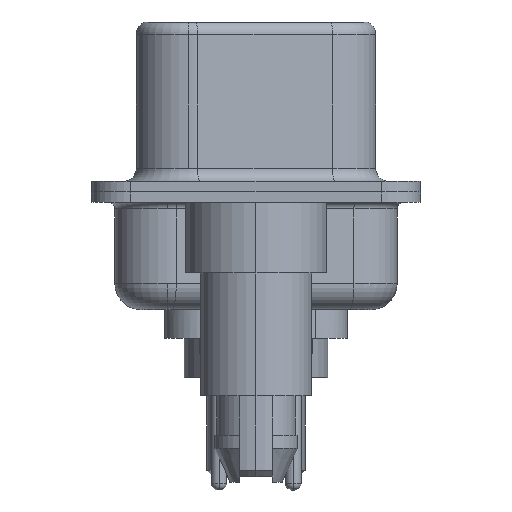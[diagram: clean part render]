
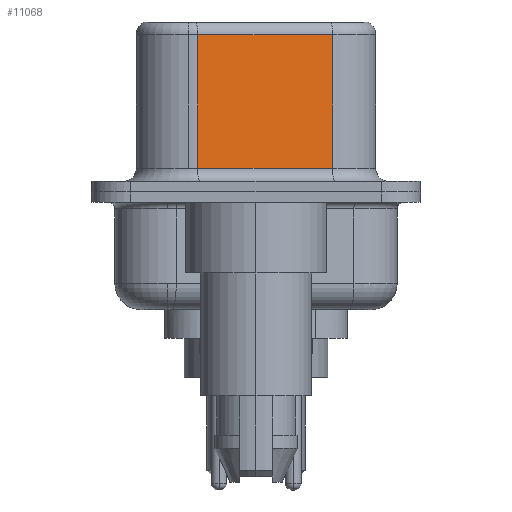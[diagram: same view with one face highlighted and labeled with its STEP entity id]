
A CAD part, left-side view. The second image highlights one B-rep face of the part: STEP entity #11068.
In plain terms, the highlighted planar face has unit normal (-0.985, -0.174, 0).
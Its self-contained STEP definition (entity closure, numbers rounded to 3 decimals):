
#732 = LINE ( 'NONE', #11536, #5417 ) ;
#1759 = LINE ( 'NONE', #18619, #18291 ) ;
#4169 = EDGE_CURVE ( 'NONE', #11080, #7311, #18189, .T. ) ;
#4664 = CARTESIAN_POINT ( 'NONE',  ( 4.565, -2.927, 0.9 ) ) ;
#5081 = DIRECTION ( 'NONE',  ( 0., 0., -1. ) ) ;
#5331 = CARTESIAN_POINT ( 'NONE',  ( 4.565, -2.927, 6.02 ) ) ;
#5417 = VECTOR ( 'NONE', #14884, 1000. ) ;
#5922 = CARTESIAN_POINT ( 'NONE',  ( 3.655, 2.233, 6.02 ) ) ;
#7033 = EDGE_CURVE ( 'NONE', #7311, #13232, #732, .T. ) ;
#7092 = CARTESIAN_POINT ( 'NONE',  ( 3.655, 2.233, 0.9 ) ) ;
#7311 = VERTEX_POINT ( 'NONE', #7092 ) ;
#7339 = EDGE_LOOP ( 'NONE', ( #12016, #11819, #9926, #9898 ) ) ;
#8549 = DIRECTION ( 'NONE',  ( 0., 0., -1. ) ) ;
#8574 = CARTESIAN_POINT ( 'NONE',  ( 3.655, 2.233, 6.52 ) ) ;
#9166 = CARTESIAN_POINT ( 'NONE',  ( 4.565, -2.927, 6.52 ) ) ;
#9392 = DIRECTION ( 'NONE',  ( 0.985, 0.174, 0. ) ) ;
#9803 = VECTOR ( 'NONE', #8549, 1000. ) ;
#9898 = ORIENTED_EDGE ( 'NONE', *, *, #7033, .T. ) ;
#9926 = ORIENTED_EDGE ( 'NONE', *, *, #4169, .T. ) ;
#11068 = ADVANCED_FACE ( 'NONE', ( #22151 ), #14391, .F. ) ;
#11080 = VERTEX_POINT ( 'NONE', #5922 ) ;
#11172 = VECTOR ( 'NONE', #15580, 1000. ) ;
#11536 = CARTESIAN_POINT ( 'NONE',  ( 4.565, -2.927, 0.9 ) ) ;
#11819 = ORIENTED_EDGE ( 'NONE', *, *, #19208, .T. ) ;
#12016 = ORIENTED_EDGE ( 'NONE', *, *, #15412, .F. ) ;
#13232 = VERTEX_POINT ( 'NONE', #4664 ) ;
#14391 = PLANE ( 'NONE',  #19053 ) ;
#14884 = DIRECTION ( 'NONE',  ( 0.174, -0.985, 0. ) ) ;
#15412 = EDGE_CURVE ( 'NONE', #18015, #13232, #1759, .T. ) ;
#15580 = DIRECTION ( 'NONE',  ( -0.174, 0.985, 0. ) ) ;
#18015 = VERTEX_POINT ( 'NONE', #21493 ) ;
#18189 = LINE ( 'NONE', #8574, #9803 ) ;
#18291 = VECTOR ( 'NONE', #5081, 1000. ) ;
#18619 = CARTESIAN_POINT ( 'NONE',  ( 4.565, -2.927, 6.52 ) ) ;
#19053 = AXIS2_PLACEMENT_3D ( 'NONE', #9166, #9392, #21118 ) ;
#19208 = EDGE_CURVE ( 'NONE', #18015, #11080, #20054, .T. ) ;
#20054 = LINE ( 'NONE', #5331, #11172 ) ;
#21118 = DIRECTION ( 'NONE',  ( -0.174, 0.985, 0. ) ) ;
#21493 = CARTESIAN_POINT ( 'NONE',  ( 4.565, -2.927, 6.02 ) ) ;
#22151 = FACE_OUTER_BOUND ( 'NONE', #7339, .T. ) ;
